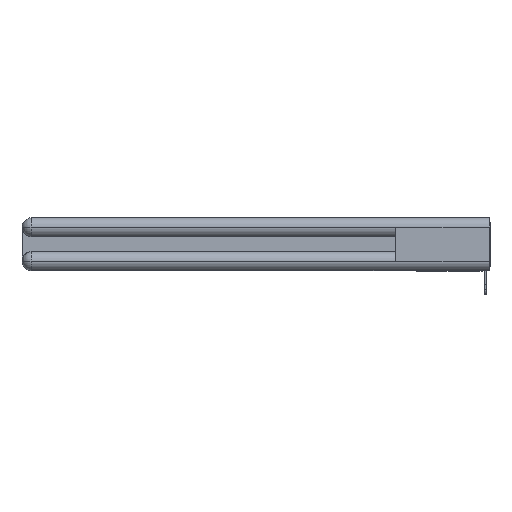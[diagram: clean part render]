
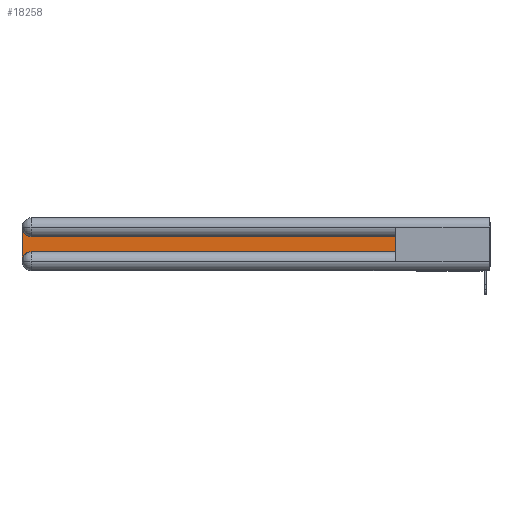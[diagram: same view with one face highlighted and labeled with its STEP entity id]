
A CAD part, left-side view. The second image highlights one B-rep face of the part: STEP entity #18258.
In plain terms, the highlighted planar face has unit normal (-1, 0, 0).
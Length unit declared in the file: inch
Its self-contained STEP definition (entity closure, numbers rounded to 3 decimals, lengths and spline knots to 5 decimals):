
#498 = CARTESIAN_POINT ( 'NONE',  ( 0.075, 2.94, -0.1225 ) ) ;
#1442 = LINE ( 'NONE', #23753, #12492 ) ;
#2696 = CIRCLE ( 'NONE', #21546, 0.06 ) ;
#2836 = DIRECTION ( 'NONE',  ( 0., 1., 0. ) ) ;
#3555 = CARTESIAN_POINT ( 'NONE',  ( 0.075, 3., -0.2175 ) ) ;
#3684 = CARTESIAN_POINT ( 'NONE',  ( 0.075, 0.6, -0.1225 ) ) ;
#3792 = ORIENTED_EDGE ( 'NONE', *, *, #26701, .T. ) ;
#4760 = VECTOR ( 'NONE', #2836, 39.37008 ) ;
#6554 = ORIENTED_EDGE ( 'NONE', *, *, #25898, .T. ) ;
#6595 = CARTESIAN_POINT ( 'NONE',  ( 0.075, 3., -0.0625 ) ) ;
#6803 = PLANE ( 'NONE',  #16220 ) ;
#7515 = VERTEX_POINT ( 'NONE', #6595 ) ;
#8517 = CIRCLE ( 'NONE', #19900, 0.06 ) ;
#8527 = CARTESIAN_POINT ( 'NONE',  ( 0.075, 2.94, -0.2175 ) ) ;
#8732 = VERTEX_POINT ( 'NONE', #8527 ) ;
#8796 = LINE ( 'NONE', #3555, #20594 ) ;
#9432 = VERTEX_POINT ( 'NONE', #24830 ) ;
#10244 = DIRECTION ( 'NONE',  ( 1., 0., 0. ) ) ;
#10407 = DIRECTION ( 'NONE',  ( 0., 0., -1. ) ) ;
#11668 = LINE ( 'NONE', #16206, #4760 ) ;
#12256 = VERTEX_POINT ( 'NONE', #3684 ) ;
#12442 = CARTESIAN_POINT ( 'NONE',  ( 0.075, 2.94, -0.2775 ) ) ;
#12492 = VECTOR ( 'NONE', #14763, 39.37008 ) ;
#13266 = ORIENTED_EDGE ( 'NONE', *, *, #14248, .T. ) ;
#13786 = DIRECTION ( 'NONE',  ( 1., 0., 0. ) ) ;
#14248 = EDGE_CURVE ( 'NONE', #12256, #25098, #11668, .T. ) ;
#14763 = DIRECTION ( 'NONE',  ( 0., 0., 1. ) ) ;
#16206 = CARTESIAN_POINT ( 'NONE',  ( 0.075, 0.6, -0.1225 ) ) ;
#16220 = AXIS2_PLACEMENT_3D ( 'NONE', #20176, #13786, #24609 ) ;
#16481 = EDGE_CURVE ( 'NONE', #8732, #22592, #17215, .T. ) ;
#16754 = CARTESIAN_POINT ( 'NONE',  ( 0.075, 2.94, -0.0625 ) ) ;
#17215 = LINE ( 'NONE', #18083, #25473 ) ;
#17434 = FACE_OUTER_BOUND ( 'NONE', #18518, .T. ) ;
#17485 = EDGE_CURVE ( 'NONE', #7515, #9432, #8796, .T. ) ;
#18083 = CARTESIAN_POINT ( 'NONE',  ( 0.075, 0.6, -0.2175 ) ) ;
#18258 = ADVANCED_FACE ( 'NONE', ( #17434 ), #6803, .F. ) ;
#18518 = EDGE_LOOP ( 'NONE', ( #13266, #6554, #19378, #3792, #24457, #23185 ) ) ;
#19048 = DIRECTION ( 'NONE',  ( 0., 0., -1. ) ) ;
#19378 = ORIENTED_EDGE ( 'NONE', *, *, #17485, .T. ) ;
#19900 = AXIS2_PLACEMENT_3D ( 'NONE', #12442, #25894, #10407 ) ;
#19966 = EDGE_CURVE ( 'NONE', #22592, #12256, #1442, .T. ) ;
#20176 = CARTESIAN_POINT ( 'NONE',  ( 0.075, 3., -0.1225 ) ) ;
#20594 = VECTOR ( 'NONE', #19048, 39.37008 ) ;
#21394 = DIRECTION ( 'NONE',  ( 0., 0., -1. ) ) ;
#21546 = AXIS2_PLACEMENT_3D ( 'NONE', #16754, #10244, #21394 ) ;
#22140 = CARTESIAN_POINT ( 'NONE',  ( 0.075, 0.6, -0.2175 ) ) ;
#22592 = VERTEX_POINT ( 'NONE', #22140 ) ;
#23185 = ORIENTED_EDGE ( 'NONE', *, *, #19966, .T. ) ;
#23753 = CARTESIAN_POINT ( 'NONE',  ( 0.075, 0.6, -0.2175 ) ) ;
#24457 = ORIENTED_EDGE ( 'NONE', *, *, #16481, .T. ) ;
#24575 = DIRECTION ( 'NONE',  ( 0., -1., 0. ) ) ;
#24609 = DIRECTION ( 'NONE',  ( 0., 0., -1. ) ) ;
#24830 = CARTESIAN_POINT ( 'NONE',  ( 0.075, 3., -0.2775 ) ) ;
#25098 = VERTEX_POINT ( 'NONE', #498 ) ;
#25473 = VECTOR ( 'NONE', #24575, 39.37008 ) ;
#25894 = DIRECTION ( 'NONE',  ( 1., 0., 0. ) ) ;
#25898 = EDGE_CURVE ( 'NONE', #25098, #7515, #2696, .T. ) ;
#26701 = EDGE_CURVE ( 'NONE', #9432, #8732, #8517, .T. ) ;
